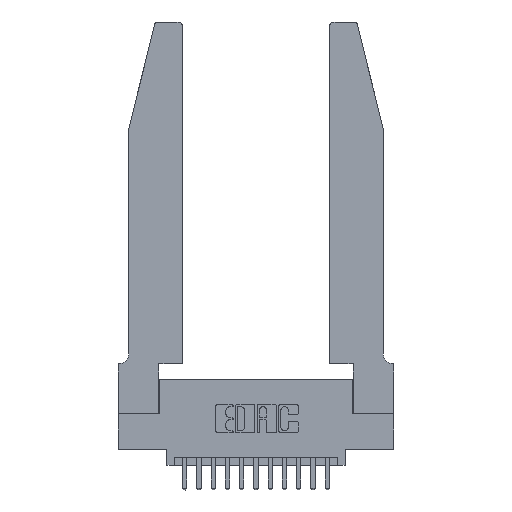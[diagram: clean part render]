
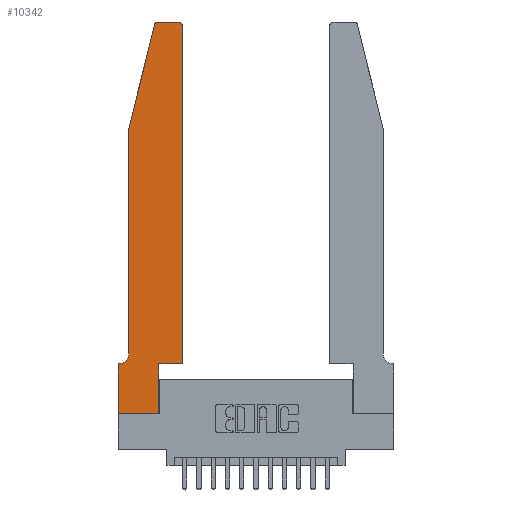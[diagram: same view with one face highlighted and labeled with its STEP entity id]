
A CAD part, top view. The second image highlights one B-rep face of the part: STEP entity #10342.
In plain terms, the highlighted planar face has unit normal (0, 0, 1).
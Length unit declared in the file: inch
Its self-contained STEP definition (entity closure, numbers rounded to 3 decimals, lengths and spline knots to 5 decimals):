
#46 = ORIENTED_EDGE ( 'NONE', *, *, #8549, .T. ) ;
#104 = CARTESIAN_POINT ( 'NONE',  ( 0.2605, 2.75, 0.37 ) ) ;
#129 = DIRECTION ( 'NONE',  ( 0., 0., 1. ) ) ;
#346 = CARTESIAN_POINT ( 'NONE',  ( 0.4205, 2.75, 0.37 ) ) ;
#796 = ORIENTED_EDGE ( 'NONE', *, *, #13554, .T. ) ;
#963 = EDGE_CURVE ( 'NONE', #12793, #12190, #1530, .T. ) ;
#1324 = DIRECTION ( 'NONE',  ( 0., 0., 1. ) ) ;
#1503 = ORIENTED_EDGE ( 'NONE', *, *, #10217, .T. ) ;
#1530 = LINE ( 'NONE', #4319, #5008 ) ;
#1554 = AXIS2_PLACEMENT_3D ( 'NONE', #2818, #129, #6986 ) ;
#1716 = CARTESIAN_POINT ( 'NONE',  ( 0.2865, 0., 0.37 ) ) ;
#1996 = VERTEX_POINT ( 'NONE', #3420 ) ;
#2179 = CARTESIAN_POINT ( 'NONE',  ( 0., 0.35, 0.37 ) ) ;
#2481 = CARTESIAN_POINT ( 'NONE',  ( 0.0755, 2., 0.37 ) ) ;
#2818 = CARTESIAN_POINT ( 'NONE',  ( 0.4205, 2.72, 0.37 ) ) ;
#3025 = VERTEX_POINT ( 'NONE', #6526 ) ;
#3158 = LINE ( 'NONE', #8530, #10686 ) ;
#3420 = CARTESIAN_POINT ( 'NONE',  ( 0.4505, 2.72, 0.37 ) ) ;
#3534 = CARTESIAN_POINT ( 'NONE',  ( 0.0055, 0.35, 0.37 ) ) ;
#3538 = VERTEX_POINT ( 'NONE', #2179 ) ;
#3587 = DIRECTION ( 'NONE',  ( 1., 0., 0. ) ) ;
#3709 = VECTOR ( 'NONE', #12525, 39.37008 ) ;
#4258 = DIRECTION ( 'NONE',  ( -1., 0., 0. ) ) ;
#4319 = CARTESIAN_POINT ( 'NONE',  ( 0., 0., 0.37 ) ) ;
#4476 = CARTESIAN_POINT ( 'NONE',  ( 0., 0.35, 0.37 ) ) ;
#4592 = DIRECTION ( 'NONE',  ( 0., 1., 0. ) ) ;
#5008 = VECTOR ( 'NONE', #3587, 39.37008 ) ;
#5050 = ORIENTED_EDGE ( 'NONE', *, *, #11124, .T. ) ;
#5294 = VECTOR ( 'NONE', #15858, 39.37008 ) ;
#5624 = LINE ( 'NONE', #12001, #9886 ) ;
#5972 = ORIENTED_EDGE ( 'NONE', *, *, #963, .T. ) ;
#6017 = VECTOR ( 'NONE', #17119, 39.37008 ) ;
#6099 = EDGE_CURVE ( 'NONE', #16643, #3538, #13236, .T. ) ;
#6104 = CIRCLE ( 'NONE', #17479, 0.07 ) ;
#6193 = ORIENTED_EDGE ( 'NONE', *, *, #6099, .T. ) ;
#6335 = LINE ( 'NONE', #104, #10808 ) ;
#6430 = CARTESIAN_POINT ( 'NONE',  ( 0.4505, 0.35, 0.37 ) ) ;
#6500 = AXIS2_PLACEMENT_3D ( 'NONE', #9557, #1324, #10941 ) ;
#6526 = CARTESIAN_POINT ( 'NONE',  ( 0.284, 2.75, 0.37 ) ) ;
#6528 = ORIENTED_EDGE ( 'NONE', *, *, #6759, .T. ) ;
#6622 = DIRECTION ( 'NONE',  ( 0., 1., 0. ) ) ;
#6759 = EDGE_CURVE ( 'NONE', #3538, #12793, #14492, .T. ) ;
#6842 = VECTOR ( 'NONE', #7382, 39.37008 ) ;
#6986 = DIRECTION ( 'NONE',  ( 1., 0., 0. ) ) ;
#7382 = DIRECTION ( 'NONE',  ( -1., 0., 0. ) ) ;
#7406 = EDGE_LOOP ( 'NONE', ( #15160, #1503, #796, #46, #13413, #6193, #6528, #5972, #5050, #10045, #7503, #13133 ) ) ;
#7503 = ORIENTED_EDGE ( 'NONE', *, *, #12541, .T. ) ;
#7810 = DIRECTION ( 'NONE',  ( 1., 0., 0. ) ) ;
#7939 = EDGE_CURVE ( 'NONE', #15764, #16643, #6104, .T. ) ;
#7961 = EDGE_CURVE ( 'NONE', #9889, #3025, #6335, .T. ) ;
#8514 = EDGE_CURVE ( 'NONE', #13909, #16945, #12919, .T. ) ;
#8530 = CARTESIAN_POINT ( 'NONE',  ( 0.2865, 0.35, 0.37 ) ) ;
#8549 = EDGE_CURVE ( 'NONE', #17821, #15764, #9294, .T. ) ;
#8619 = CARTESIAN_POINT ( 'NONE',  ( 0., 0., 0.37 ) ) ;
#9095 = CARTESIAN_POINT ( 'NONE',  ( 0., 0., 0.37 ) ) ;
#9294 = LINE ( 'NONE', #2481, #3709 ) ;
#9557 = CARTESIAN_POINT ( 'NONE',  ( 0.284, 2.72, 0.37 ) ) ;
#9581 = CARTESIAN_POINT ( 'NONE',  ( 0.0055, 0.42, 0.37 ) ) ;
#9832 = DIRECTION ( 'NONE',  ( 1., 0., 0. ) ) ;
#9886 = VECTOR ( 'NONE', #6622, 39.37008 ) ;
#9889 = VERTEX_POINT ( 'NONE', #346 ) ;
#10045 = ORIENTED_EDGE ( 'NONE', *, *, #8514, .T. ) ;
#10092 = CARTESIAN_POINT ( 'NONE',  ( 0.2865, 0.35, 0.37 ) ) ;
#10217 = EDGE_CURVE ( 'NONE', #3025, #16827, #13718, .T. ) ;
#10342 = ADVANCED_FACE ( 'NONE', ( #10725 ), #15317, .T. ) ;
#10686 = VECTOR ( 'NONE', #4592, 39.37008 ) ;
#10725 = FACE_OUTER_BOUND ( 'NONE', #7406, .T. ) ;
#10808 = VECTOR ( 'NONE', #12400, 39.37008 ) ;
#10941 = DIRECTION ( 'NONE',  ( 1., 0., 0. ) ) ;
#11013 = CIRCLE ( 'NONE', #1554, 0.03 ) ;
#11021 = DIRECTION ( 'NONE',  ( 0., 0., -1. ) ) ;
#11124 = EDGE_CURVE ( 'NONE', #12190, #13909, #3158, .T. ) ;
#11181 = CARTESIAN_POINT ( 'NONE',  ( 0.0755, 0.42, 0.37 ) ) ;
#11659 = EDGE_CURVE ( 'NONE', #1996, #9889, #11013, .T. ) ;
#12001 = CARTESIAN_POINT ( 'NONE',  ( 0.4505, 0.35, 0.37 ) ) ;
#12190 = VERTEX_POINT ( 'NONE', #1716 ) ;
#12400 = DIRECTION ( 'NONE',  ( -1., 0., 0. ) ) ;
#12525 = DIRECTION ( 'NONE',  ( 0., -1., 0. ) ) ;
#12541 = EDGE_CURVE ( 'NONE', #16945, #1996, #5624, .T. ) ;
#12696 = VECTOR ( 'NONE', #7810, 39.37008 ) ;
#12793 = VERTEX_POINT ( 'NONE', #8619 ) ;
#12919 = LINE ( 'NONE', #6430, #12696 ) ;
#13133 = ORIENTED_EDGE ( 'NONE', *, *, #11659, .T. ) ;
#13236 = LINE ( 'NONE', #14159, #6842 ) ;
#13413 = ORIENTED_EDGE ( 'NONE', *, *, #7939, .T. ) ;
#13554 = EDGE_CURVE ( 'NONE', #16827, #17821, #16324, .T. ) ;
#13718 = CIRCLE ( 'NONE', #6500, 0.03 ) ;
#13909 = VERTEX_POINT ( 'NONE', #10092 ) ;
#14159 = CARTESIAN_POINT ( 'NONE',  ( 0.0755, 0.35, 0.37 ) ) ;
#14163 = CARTESIAN_POINT ( 'NONE',  ( 0.0755, 2., 0.37 ) ) ;
#14180 = CARTESIAN_POINT ( 'NONE',  ( 0.0755, 2., 0.37 ) ) ;
#14492 = LINE ( 'NONE', #9095, #5294 ) ;
#15160 = ORIENTED_EDGE ( 'NONE', *, *, #7961, .T. ) ;
#15317 = PLANE ( 'NONE',  #16008 ) ;
#15764 = VERTEX_POINT ( 'NONE', #11181 ) ;
#15858 = DIRECTION ( 'NONE',  ( 0., -1., 0. ) ) ;
#16008 = AXIS2_PLACEMENT_3D ( 'NONE', #4476, #16663, #9832 ) ;
#16324 = LINE ( 'NONE', #14180, #6017 ) ;
#16478 = CARTESIAN_POINT ( 'NONE',  ( 0.25487, 2.72718, 0.37 ) ) ;
#16643 = VERTEX_POINT ( 'NONE', #3534 ) ;
#16663 = DIRECTION ( 'NONE',  ( 0., 0., 1. ) ) ;
#16712 = CARTESIAN_POINT ( 'NONE',  ( 0.4505, 0.35, 0.37 ) ) ;
#16827 = VERTEX_POINT ( 'NONE', #16478 ) ;
#16945 = VERTEX_POINT ( 'NONE', #16712 ) ;
#17119 = DIRECTION ( 'NONE',  ( -0.239, -0.971, 0. ) ) ;
#17479 = AXIS2_PLACEMENT_3D ( 'NONE', #9581, #11021, #4258 ) ;
#17821 = VERTEX_POINT ( 'NONE', #14163 ) ;
